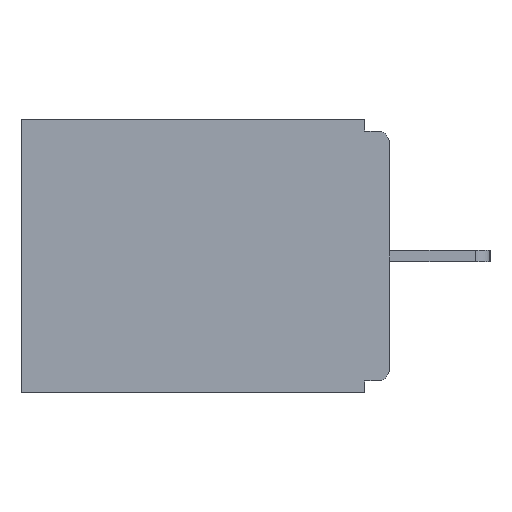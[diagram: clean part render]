
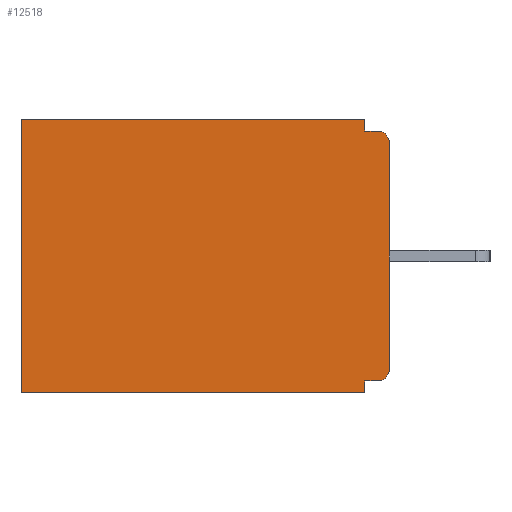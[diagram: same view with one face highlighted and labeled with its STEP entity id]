
A CAD part, left-side view. The second image highlights one B-rep face of the part: STEP entity #12518.
In plain terms, the highlighted planar face has unit normal (-1, 0, 0).
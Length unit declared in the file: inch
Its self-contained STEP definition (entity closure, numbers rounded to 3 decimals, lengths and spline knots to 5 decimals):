
#42 = VERTEX_POINT ( 'NONE', #22347 ) ;
#154 = LINE ( 'NONE', #7434, #18581 ) ;
#511 = VERTEX_POINT ( 'NONE', #792 ) ;
#792 = CARTESIAN_POINT ( 'NONE',  ( 0.298, 0.015, -0.015 ) ) ;
#1149 = ORIENTED_EDGE ( 'NONE', *, *, #22643, .F. ) ;
#1628 = EDGE_LOOP ( 'NONE', ( #21207, #3824, #13968, #22792, #15036, #1149, #20442, #12058, #17163, #22534 ) ) ;
#1795 = VECTOR ( 'NONE', #2592, 39.37008 ) ;
#1944 = CARTESIAN_POINT ( 'NONE',  ( 0.298, 0., -0.015 ) ) ;
#2340 = DIRECTION ( 'NONE',  ( -1., 0., 0. ) ) ;
#2537 = CARTESIAN_POINT ( 'NONE',  ( 0.298, 0.031, -0.328 ) ) ;
#2569 = PLANE ( 'NONE',  #11822 ) ;
#2592 = DIRECTION ( 'NONE',  ( 0., -1., 0. ) ) ;
#3824 = ORIENTED_EDGE ( 'NONE', *, *, #10694, .F. ) ;
#4221 = CARTESIAN_POINT ( 'NONE',  ( 0.298, 0.015, -0.328 ) ) ;
#4356 = VERTEX_POINT ( 'NONE', #17736 ) ;
#4645 = VERTEX_POINT ( 'NONE', #15141 ) ;
#5211 = EDGE_CURVE ( 'NONE', #10609, #12180, #154, .T. ) ;
#5290 = EDGE_CURVE ( 'NONE', #12180, #4356, #12486, .T. ) ;
#5966 = DIRECTION ( 'NONE',  ( 0., 1., 0. ) ) ;
#6059 = VECTOR ( 'NONE', #6815, 39.37008 ) ;
#6354 = CIRCLE ( 'NONE', #20737, 0.015 ) ;
#6708 = VECTOR ( 'NONE', #19938, 39.37008 ) ;
#6815 = DIRECTION ( 'NONE',  ( 0., 1., 0. ) ) ;
#7305 = CARTESIAN_POINT ( 'NONE',  ( 0.298, 0., 0. ) ) ;
#7360 = LINE ( 'NONE', #7305, #11013 ) ;
#7434 = CARTESIAN_POINT ( 'NONE',  ( 0.298, 0., 0. ) ) ;
#7550 = VERTEX_POINT ( 'NONE', #17900 ) ;
#8211 = DIRECTION ( 'NONE',  ( 0., 0., -1. ) ) ;
#10609 = VERTEX_POINT ( 'NONE', #18107 ) ;
#10694 = EDGE_CURVE ( 'NONE', #13221, #511, #20463, .T. ) ;
#10863 = LINE ( 'NONE', #17434, #14361 ) ;
#10886 = LINE ( 'NONE', #17293, #6059 ) ;
#11013 = VECTOR ( 'NONE', #20974, 39.37008 ) ;
#11040 = DIRECTION ( 'NONE',  ( -1., 0., 0. ) ) ;
#11367 = AXIS2_PLACEMENT_3D ( 'NONE', #21080, #11040, #22777 ) ;
#11428 = VECTOR ( 'NONE', #14120, 39.37008 ) ;
#11446 = CIRCLE ( 'NONE', #11367, 0.015 ) ;
#11494 = LINE ( 'NONE', #21606, #6708 ) ;
#11656 = CARTESIAN_POINT ( 'NONE',  ( 0.298, 0., 0. ) ) ;
#11822 = AXIS2_PLACEMENT_3D ( 'NONE', #11656, #18470, #8211 ) ;
#12058 = ORIENTED_EDGE ( 'NONE', *, *, #15331, .F. ) ;
#12180 = VERTEX_POINT ( 'NONE', #19390 ) ;
#12486 = LINE ( 'NONE', #18515, #11428 ) ;
#12518 = ADVANCED_FACE ( 'NONE', ( #21979 ), #2569, .F. ) ;
#13181 = CARTESIAN_POINT ( 'NONE',  ( 0.298, 0.015, -0.03 ) ) ;
#13221 = VERTEX_POINT ( 'NONE', #16612 ) ;
#13280 = VERTEX_POINT ( 'NONE', #2537 ) ;
#13968 = ORIENTED_EDGE ( 'NONE', *, *, #17613, .F. ) ;
#14041 = EDGE_CURVE ( 'NONE', #42, #511, #6354, .T. ) ;
#14120 = DIRECTION ( 'NONE',  ( 0., 0., -1. ) ) ;
#14361 = VECTOR ( 'NONE', #18983, 39.37008 ) ;
#14602 = CARTESIAN_POINT ( 'NONE',  ( 0.298, 0.031, -0.343 ) ) ;
#14745 = LINE ( 'NONE', #14602, #18648 ) ;
#14935 = DIRECTION ( 'NONE',  ( 0., 0., -1. ) ) ;
#15036 = ORIENTED_EDGE ( 'NONE', *, *, #5290, .T. ) ;
#15141 = CARTESIAN_POINT ( 'NONE',  ( 0.298, 0., -0.313 ) ) ;
#15331 = EDGE_CURVE ( 'NONE', #20422, #13280, #10886, .T. ) ;
#16337 = EDGE_CURVE ( 'NONE', #20422, #4645, #11446, .T. ) ;
#16612 = CARTESIAN_POINT ( 'NONE',  ( 0.298, 0.031, -0.015 ) ) ;
#17163 = ORIENTED_EDGE ( 'NONE', *, *, #16337, .T. ) ;
#17293 = CARTESIAN_POINT ( 'NONE',  ( 0.298, 0., -0.328 ) ) ;
#17434 = CARTESIAN_POINT ( 'NONE',  ( 0.298, 0.031, -0.343 ) ) ;
#17613 = EDGE_CURVE ( 'NONE', #10609, #13221, #10863, .T. ) ;
#17736 = CARTESIAN_POINT ( 'NONE',  ( 0.298, 0.46, -0.343 ) ) ;
#17900 = CARTESIAN_POINT ( 'NONE',  ( 0.298, 0.031, -0.343 ) ) ;
#18107 = CARTESIAN_POINT ( 'NONE',  ( 0.298, 0.031, 0. ) ) ;
#18470 = DIRECTION ( 'NONE',  ( 1., 0., 0. ) ) ;
#18515 = CARTESIAN_POINT ( 'NONE',  ( 0.298, 0.46, 0. ) ) ;
#18581 = VECTOR ( 'NONE', #5966, 39.37008 ) ;
#18648 = VECTOR ( 'NONE', #19590, 39.37008 ) ;
#18983 = DIRECTION ( 'NONE',  ( 0., 0., -1. ) ) ;
#19390 = CARTESIAN_POINT ( 'NONE',  ( 0.298, 0.46, 0. ) ) ;
#19590 = DIRECTION ( 'NONE',  ( 0., 0., -1. ) ) ;
#19938 = DIRECTION ( 'NONE',  ( 0., 1., 0. ) ) ;
#20422 = VERTEX_POINT ( 'NONE', #4221 ) ;
#20442 = ORIENTED_EDGE ( 'NONE', *, *, #22466, .F. ) ;
#20463 = LINE ( 'NONE', #1944, #1795 ) ;
#20737 = AXIS2_PLACEMENT_3D ( 'NONE', #13181, #2340, #14935 ) ;
#20823 = EDGE_CURVE ( 'NONE', #42, #4645, #7360, .T. ) ;
#20974 = DIRECTION ( 'NONE',  ( 0., 0., -1. ) ) ;
#21080 = CARTESIAN_POINT ( 'NONE',  ( 0.298, 0.015, -0.313 ) ) ;
#21207 = ORIENTED_EDGE ( 'NONE', *, *, #14041, .T. ) ;
#21606 = CARTESIAN_POINT ( 'NONE',  ( 0.298, 0., -0.343 ) ) ;
#21979 = FACE_OUTER_BOUND ( 'NONE', #1628, .T. ) ;
#22347 = CARTESIAN_POINT ( 'NONE',  ( 0.298, 0., -0.03 ) ) ;
#22466 = EDGE_CURVE ( 'NONE', #13280, #7550, #14745, .T. ) ;
#22534 = ORIENTED_EDGE ( 'NONE', *, *, #20823, .F. ) ;
#22643 = EDGE_CURVE ( 'NONE', #7550, #4356, #11494, .T. ) ;
#22777 = DIRECTION ( 'NONE',  ( 0., 0., -1. ) ) ;
#22792 = ORIENTED_EDGE ( 'NONE', *, *, #5211, .T. ) ;
